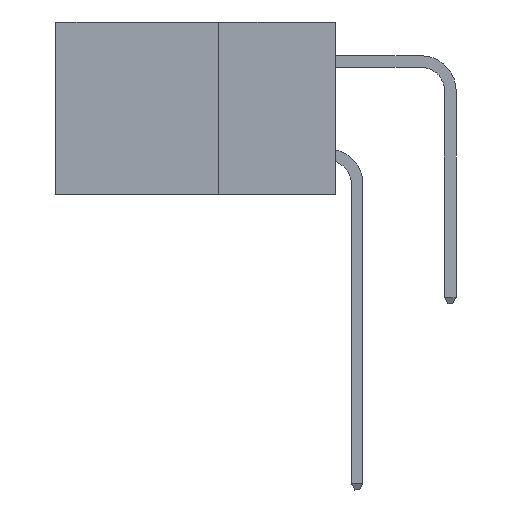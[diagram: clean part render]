
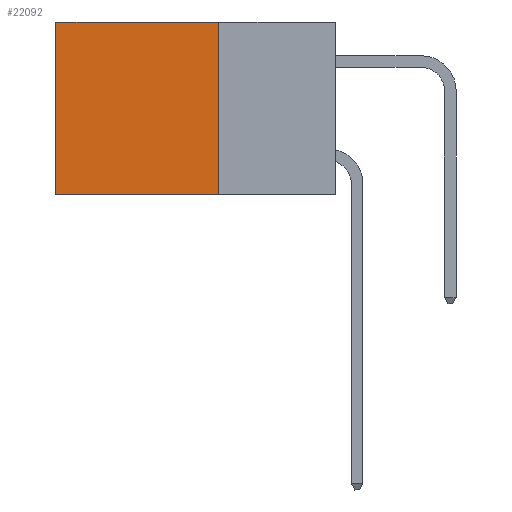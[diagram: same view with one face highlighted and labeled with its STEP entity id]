
A CAD part, left-side view. The second image highlights one B-rep face of the part: STEP entity #22092.
In plain terms, the highlighted planar face has unit normal (-1, 0, 0).
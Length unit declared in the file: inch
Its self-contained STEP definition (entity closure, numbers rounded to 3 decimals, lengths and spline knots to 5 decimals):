
#1459 = ORIENTED_EDGE ( 'NONE', *, *, #19824, .F. ) ;
#1509 = LINE ( 'NONE', #22284, #24529 ) ;
#1631 = VECTOR ( 'NONE', #20584, 39.37008 ) ;
#2719 = CARTESIAN_POINT ( 'NONE',  ( 0.2875, 0.6, -0.37 ) ) ;
#2734 = PLANE ( 'NONE',  #27328 ) ;
#3548 = DIRECTION ( 'NONE',  ( 0., 0., -1. ) ) ;
#5063 = DIRECTION ( 'NONE',  ( 1., 0., 0. ) ) ;
#5485 = VERTEX_POINT ( 'NONE', #5861 ) ;
#5688 = CARTESIAN_POINT ( 'NONE',  ( 0.2875, 0.6, 0. ) ) ;
#5861 = CARTESIAN_POINT ( 'NONE',  ( 0.2875, 0.25, -0.37 ) ) ;
#6941 = CARTESIAN_POINT ( 'NONE',  ( 0.2875, 0.25, 0. ) ) ;
#7339 = ORIENTED_EDGE ( 'NONE', *, *, #19257, .F. ) ;
#7656 = ORIENTED_EDGE ( 'NONE', *, *, #15325, .T. ) ;
#9797 = CARTESIAN_POINT ( 'NONE',  ( 0.2875, 0.25, 0. ) ) ;
#9969 = VECTOR ( 'NONE', #18723, 39.37008 ) ;
#11852 = LINE ( 'NONE', #14069, #9969 ) ;
#12602 = VERTEX_POINT ( 'NONE', #2719 ) ;
#14069 = CARTESIAN_POINT ( 'NONE',  ( 0.2875, 0.25, 0. ) ) ;
#15325 = EDGE_CURVE ( 'NONE', #22351, #12602, #16330, .T. ) ;
#16239 = VECTOR ( 'NONE', #3548, 39.37008 ) ;
#16330 = LINE ( 'NONE', #24578, #1631 ) ;
#18723 = DIRECTION ( 'NONE',  ( 0., 1., 0. ) ) ;
#18838 = VERTEX_POINT ( 'NONE', #6941 ) ;
#19257 = EDGE_CURVE ( 'NONE', #18838, #5485, #22301, .T. ) ;
#19824 = EDGE_CURVE ( 'NONE', #5485, #12602, #1509, .T. ) ;
#20584 = DIRECTION ( 'NONE',  ( 0., 0., -1. ) ) ;
#21012 = FACE_OUTER_BOUND ( 'NONE', #21691, .T. ) ;
#21691 = EDGE_LOOP ( 'NONE', ( #7656, #1459, #7339, #21707 ) ) ;
#21707 = ORIENTED_EDGE ( 'NONE', *, *, #27020, .T. ) ;
#22092 = ADVANCED_FACE ( 'NONE', ( #21012 ), #2734, .F. ) ;
#22284 = CARTESIAN_POINT ( 'NONE',  ( 0.2875, 0.25, -0.37 ) ) ;
#22301 = LINE ( 'NONE', #27404, #16239 ) ;
#22351 = VERTEX_POINT ( 'NONE', #5688 ) ;
#24529 = VECTOR ( 'NONE', #24937, 39.37008 ) ;
#24578 = CARTESIAN_POINT ( 'NONE',  ( 0.2875, 0.6, 0. ) ) ;
#24937 = DIRECTION ( 'NONE',  ( 0., 1., 0. ) ) ;
#27020 = EDGE_CURVE ( 'NONE', #18838, #22351, #11852, .T. ) ;
#27328 = AXIS2_PLACEMENT_3D ( 'NONE', #9797, #5063, #29441 ) ;
#27404 = CARTESIAN_POINT ( 'NONE',  ( 0.2875, 0.25, 0. ) ) ;
#29441 = DIRECTION ( 'NONE',  ( 0., 0., -1. ) ) ;
